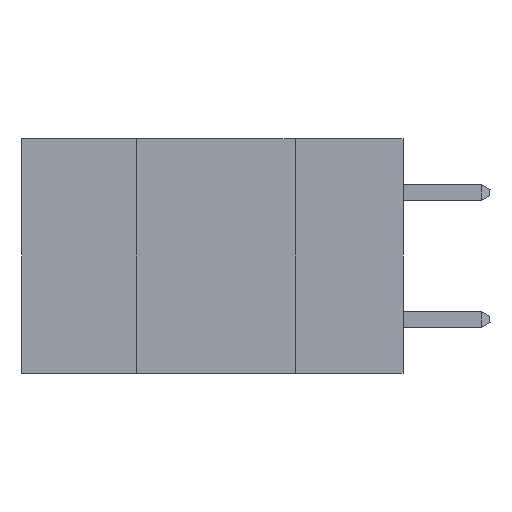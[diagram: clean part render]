
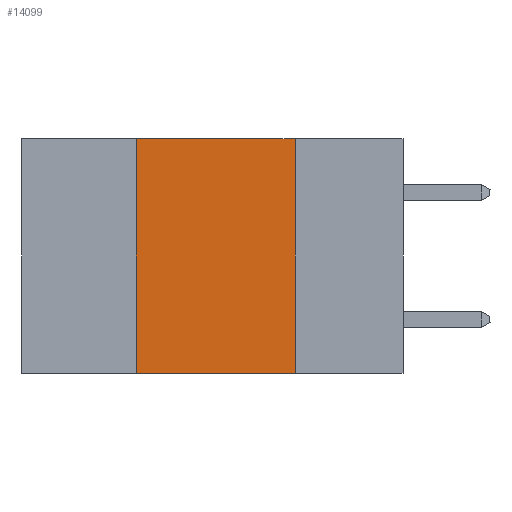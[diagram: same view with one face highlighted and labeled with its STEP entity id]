
A CAD part, left-side view. The second image highlights one B-rep face of the part: STEP entity #14099.
In plain terms, the highlighted planar face has unit normal (-1, 0, 0).
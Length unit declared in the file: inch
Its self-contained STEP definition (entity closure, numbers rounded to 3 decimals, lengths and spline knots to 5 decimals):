
#688 = DIRECTION ( 'NONE',  ( 0., 0., -1. ) ) ;
#1349 = LINE ( 'NONE', #7464, #20117 ) ;
#2583 = CARTESIAN_POINT ( 'NONE',  ( 0., 0.6, 0. ) ) ;
#3241 = CARTESIAN_POINT ( 'NONE',  ( 0., 0.42, 0. ) ) ;
#3880 = DIRECTION ( 'NONE',  ( 0., 0., 1. ) ) ;
#6293 = DIRECTION ( 'NONE',  ( 0., -1., 0. ) ) ;
#6488 = VECTOR ( 'NONE', #7424, 39.37008 ) ;
#6932 = ORIENTED_EDGE ( 'NONE', *, *, #15983, .T. ) ;
#7424 = DIRECTION ( 'NONE',  ( 0., -1., 0. ) ) ;
#7464 = CARTESIAN_POINT ( 'NONE',  ( 0., 0.42, 0. ) ) ;
#8408 = VECTOR ( 'NONE', #10014, 39.37008 ) ;
#9081 = VECTOR ( 'NONE', #6293, 39.37008 ) ;
#9194 = EDGE_CURVE ( 'NONE', #20397, #22638, #1349, .T. ) ;
#10014 = DIRECTION ( 'NONE',  ( 0., 0., -1. ) ) ;
#10239 = LINE ( 'NONE', #2583, #9081 ) ;
#11379 = CARTESIAN_POINT ( 'NONE',  ( 0., 0.6, 0. ) ) ;
#11698 = DIRECTION ( 'NONE',  ( 1., 0., 0. ) ) ;
#11945 = EDGE_CURVE ( 'NONE', #22154, #19499, #22587, .T. ) ;
#12076 = ORIENTED_EDGE ( 'NONE', *, *, #9194, .F. ) ;
#12731 = AXIS2_PLACEMENT_3D ( 'NONE', #11379, #11698, #688 ) ;
#13673 = LINE ( 'NONE', #23680, #6488 ) ;
#14099 = ADVANCED_FACE ( 'NONE', ( #23077 ), #17124, .F. ) ;
#15983 = EDGE_CURVE ( 'NONE', #20397, #19499, #13673, .T. ) ;
#17124 = PLANE ( 'NONE',  #12731 ) ;
#17700 = ORIENTED_EDGE ( 'NONE', *, *, #21027, .F. ) ;
#18032 = EDGE_LOOP ( 'NONE', ( #21534, #17700, #12076, #6932 ) ) ;
#18255 = CARTESIAN_POINT ( 'NONE',  ( 0., 0.17, 0. ) ) ;
#19499 = VERTEX_POINT ( 'NONE', #22411 ) ;
#20117 = VECTOR ( 'NONE', #3880, 39.37008 ) ;
#20397 = VERTEX_POINT ( 'NONE', #21181 ) ;
#21027 = EDGE_CURVE ( 'NONE', #22638, #22154, #10239, .T. ) ;
#21115 = CARTESIAN_POINT ( 'NONE',  ( 0., 0.17, 0. ) ) ;
#21181 = CARTESIAN_POINT ( 'NONE',  ( 0., 0.42, -0.37 ) ) ;
#21534 = ORIENTED_EDGE ( 'NONE', *, *, #11945, .F. ) ;
#22154 = VERTEX_POINT ( 'NONE', #18255 ) ;
#22411 = CARTESIAN_POINT ( 'NONE',  ( 0., 0.17, -0.37 ) ) ;
#22587 = LINE ( 'NONE', #21115, #8408 ) ;
#22638 = VERTEX_POINT ( 'NONE', #3241 ) ;
#23077 = FACE_OUTER_BOUND ( 'NONE', #18032, .T. ) ;
#23680 = CARTESIAN_POINT ( 'NONE',  ( 0., 0.6, -0.37 ) ) ;
